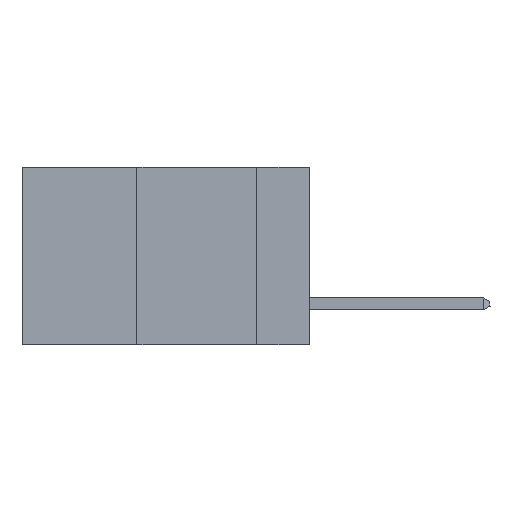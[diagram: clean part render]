
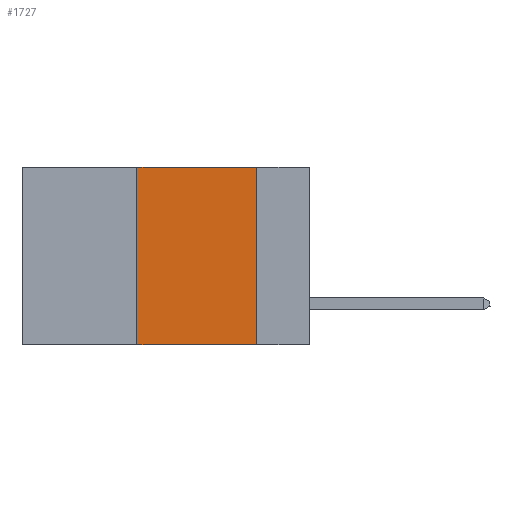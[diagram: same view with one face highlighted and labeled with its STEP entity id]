
A CAD part, left-side view. The second image highlights one B-rep face of the part: STEP entity #1727.
In plain terms, the highlighted planar face has unit normal (-1, 0, 0).
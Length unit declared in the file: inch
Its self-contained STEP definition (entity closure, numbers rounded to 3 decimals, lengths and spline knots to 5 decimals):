
#53 = CARTESIAN_POINT ( 'NONE',  ( 0., 0.11, 0. ) ) ;
#507 = CARTESIAN_POINT ( 'NONE',  ( 0., 0.36, 0. ) ) ;
#894 = EDGE_CURVE ( 'NONE', #11593, #11351, #23596, .T. ) ;
#1727 = ADVANCED_FACE ( 'NONE', ( #15580 ), #11412, .F. ) ;
#1778 = EDGE_LOOP ( 'NONE', ( #4291, #21567, #6332, #14999 ) ) ;
#3862 = EDGE_CURVE ( 'NONE', #11351, #20434, #23710, .T. ) ;
#4291 = ORIENTED_EDGE ( 'NONE', *, *, #15977, .F. ) ;
#5395 = VECTOR ( 'NONE', #21121, 39.37008 ) ;
#5722 = DIRECTION ( 'NONE',  ( 1., 0., 0. ) ) ;
#6332 = ORIENTED_EDGE ( 'NONE', *, *, #894, .F. ) ;
#6479 = LINE ( 'NONE', #21348, #13572 ) ;
#8377 = VECTOR ( 'NONE', #21613, 39.37008 ) ;
#8975 = LINE ( 'NONE', #14006, #8377 ) ;
#11351 = VERTEX_POINT ( 'NONE', #23681 ) ;
#11412 = PLANE ( 'NONE',  #19498 ) ;
#11593 = VERTEX_POINT ( 'NONE', #24061 ) ;
#11830 = CARTESIAN_POINT ( 'NONE',  ( 0., 0.11, -0.37 ) ) ;
#12746 = CARTESIAN_POINT ( 'NONE',  ( 0., 0.6, 0. ) ) ;
#13572 = VECTOR ( 'NONE', #21581, 39.37008 ) ;
#14006 = CARTESIAN_POINT ( 'NONE',  ( 0., 0.11, 0. ) ) ;
#14999 = ORIENTED_EDGE ( 'NONE', *, *, #19518, .T. ) ;
#15458 = VECTOR ( 'NONE', #20357, 39.37008 ) ;
#15580 = FACE_OUTER_BOUND ( 'NONE', #1778, .T. ) ;
#15977 = EDGE_CURVE ( 'NONE', #20434, #18857, #8975, .T. ) ;
#16877 = CARTESIAN_POINT ( 'NONE',  ( 0., 0.6, 0. ) ) ;
#18857 = VERTEX_POINT ( 'NONE', #11830 ) ;
#19498 = AXIS2_PLACEMENT_3D ( 'NONE', #16877, #5722, #20798 ) ;
#19518 = EDGE_CURVE ( 'NONE', #11593, #18857, #6479, .T. ) ;
#20357 = DIRECTION ( 'NONE',  ( 0., -1., 0. ) ) ;
#20434 = VERTEX_POINT ( 'NONE', #53 ) ;
#20798 = DIRECTION ( 'NONE',  ( 0., 0., -1. ) ) ;
#21121 = DIRECTION ( 'NONE',  ( 0., 0., 1. ) ) ;
#21348 = CARTESIAN_POINT ( 'NONE',  ( 0., 0.6, -0.37 ) ) ;
#21567 = ORIENTED_EDGE ( 'NONE', *, *, #3862, .F. ) ;
#21581 = DIRECTION ( 'NONE',  ( 0., -1., 0. ) ) ;
#21613 = DIRECTION ( 'NONE',  ( 0., 0., -1. ) ) ;
#23596 = LINE ( 'NONE', #507, #5395 ) ;
#23681 = CARTESIAN_POINT ( 'NONE',  ( 0., 0.36, 0. ) ) ;
#23710 = LINE ( 'NONE', #12746, #15458 ) ;
#24061 = CARTESIAN_POINT ( 'NONE',  ( 0., 0.36, -0.37 ) ) ;
